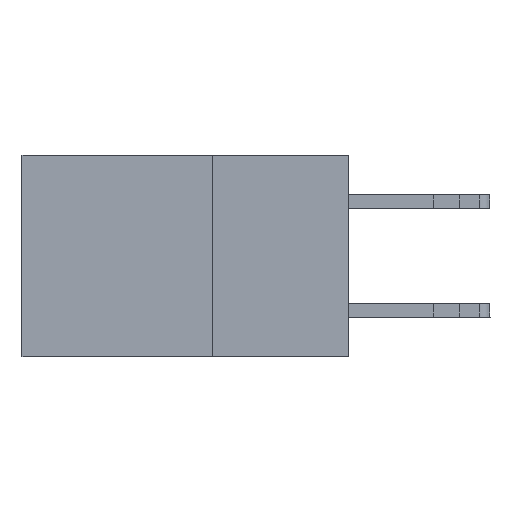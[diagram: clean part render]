
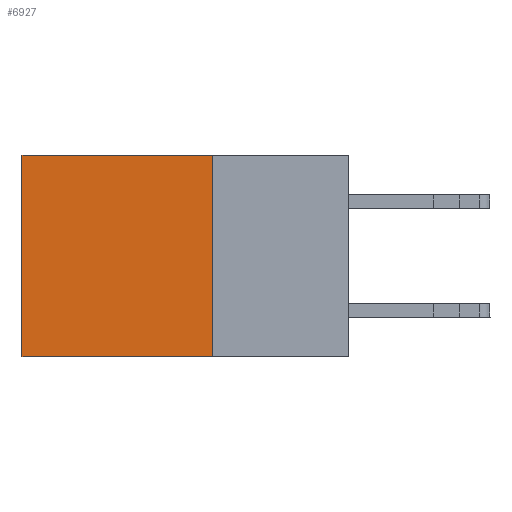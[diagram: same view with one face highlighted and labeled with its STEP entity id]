
A CAD part, left-side view. The second image highlights one B-rep face of the part: STEP entity #6927.
In plain terms, the highlighted planar face has unit normal (-1, 0, 0).
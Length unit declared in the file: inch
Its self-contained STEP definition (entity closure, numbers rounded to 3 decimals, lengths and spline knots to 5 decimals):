
#629 = CARTESIAN_POINT ( 'NONE',  ( 0.298, 0.25, 0. ) ) ;
#825 = AXIS2_PLACEMENT_3D ( 'NONE', #2948, #1987, #5634 ) ;
#898 = DIRECTION ( 'NONE',  ( 0., 0., -1. ) ) ;
#1168 = VECTOR ( 'NONE', #8485, 39.37008 ) ;
#1424 = CARTESIAN_POINT ( 'NONE',  ( 0.298, 0.25, 0. ) ) ;
#1987 = DIRECTION ( 'NONE',  ( 1., 0., 0. ) ) ;
#2049 = VECTOR ( 'NONE', #898, 39.37008 ) ;
#2470 = VECTOR ( 'NONE', #5724, 39.37008 ) ;
#2890 = VERTEX_POINT ( 'NONE', #11456 ) ;
#2948 = CARTESIAN_POINT ( 'NONE',  ( 0.298, 0.25, 0. ) ) ;
#3207 = EDGE_CURVE ( 'NONE', #9983, #2890, #11428, .T. ) ;
#3489 = LINE ( 'NONE', #4556, #2049 ) ;
#3832 = CARTESIAN_POINT ( 'NONE',  ( 0.298, 0.25, 0. ) ) ;
#4132 = VECTOR ( 'NONE', #7155, 39.37008 ) ;
#4556 = CARTESIAN_POINT ( 'NONE',  ( 0.298, 0.6, 0. ) ) ;
#4693 = CARTESIAN_POINT ( 'NONE',  ( 0.298, 0.6, -0.37 ) ) ;
#4714 = EDGE_CURVE ( 'NONE', #9983, #7060, #10669, .T. ) ;
#4888 = LINE ( 'NONE', #10190, #2470 ) ;
#5634 = DIRECTION ( 'NONE',  ( 0., 0., -1. ) ) ;
#5724 = DIRECTION ( 'NONE',  ( 0., 1., 0. ) ) ;
#6227 = FACE_OUTER_BOUND ( 'NONE', #7166, .T. ) ;
#6927 = ADVANCED_FACE ( 'NONE', ( #6227 ), #7480, .F. ) ;
#7060 = VERTEX_POINT ( 'NONE', #10457 ) ;
#7155 = DIRECTION ( 'NONE',  ( 0., 1., 0. ) ) ;
#7166 = EDGE_LOOP ( 'NONE', ( #8192, #9618, #11358, #10400 ) ) ;
#7351 = VERTEX_POINT ( 'NONE', #4693 ) ;
#7480 = PLANE ( 'NONE',  #825 ) ;
#7935 = EDGE_CURVE ( 'NONE', #7060, #7351, #3489, .T. ) ;
#8192 = ORIENTED_EDGE ( 'NONE', *, *, #7935, .T. ) ;
#8485 = DIRECTION ( 'NONE',  ( 0., 0., -1. ) ) ;
#8927 = EDGE_CURVE ( 'NONE', #2890, #7351, #4888, .T. ) ;
#9618 = ORIENTED_EDGE ( 'NONE', *, *, #8927, .F. ) ;
#9983 = VERTEX_POINT ( 'NONE', #1424 ) ;
#10190 = CARTESIAN_POINT ( 'NONE',  ( 0.298, 0.25, -0.37 ) ) ;
#10400 = ORIENTED_EDGE ( 'NONE', *, *, #4714, .T. ) ;
#10457 = CARTESIAN_POINT ( 'NONE',  ( 0.298, 0.6, 0. ) ) ;
#10669 = LINE ( 'NONE', #629, #4132 ) ;
#11358 = ORIENTED_EDGE ( 'NONE', *, *, #3207, .F. ) ;
#11428 = LINE ( 'NONE', #3832, #1168 ) ;
#11456 = CARTESIAN_POINT ( 'NONE',  ( 0.298, 0.25, -0.37 ) ) ;
